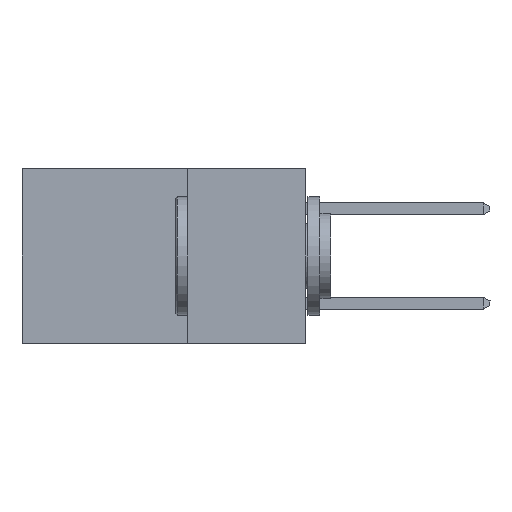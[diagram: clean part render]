
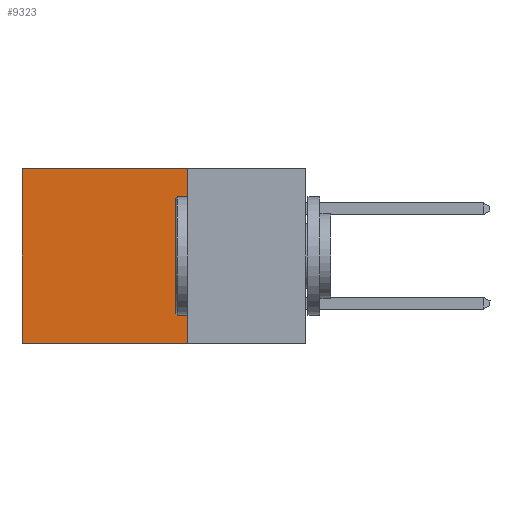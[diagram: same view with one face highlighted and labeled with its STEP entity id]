
A CAD part, left-side view. The second image highlights one B-rep face of the part: STEP entity #9323.
In plain terms, the highlighted planar face has unit normal (-1, 0, 0).
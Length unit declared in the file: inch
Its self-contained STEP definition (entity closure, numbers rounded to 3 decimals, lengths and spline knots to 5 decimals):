
#519 = LINE ( 'NONE', #17315, #11188 ) ;
#1501 = CARTESIAN_POINT ( 'NONE',  ( 0.298, 0.6, 0. ) ) ;
#3289 = CARTESIAN_POINT ( 'NONE',  ( 0.298, 0.25, 0. ) ) ;
#3666 = EDGE_CURVE ( 'NONE', #12631, #19099, #19870, .T. ) ;
#4229 = DIRECTION ( 'NONE',  ( 0., 1., 0. ) ) ;
#4754 = EDGE_CURVE ( 'NONE', #11919, #13870, #11239, .T. ) ;
#5230 = CARTESIAN_POINT ( 'NONE',  ( 0.298, 0.25, 0. ) ) ;
#5667 = FACE_OUTER_BOUND ( 'NONE', #6035, .T. ) ;
#5844 = CARTESIAN_POINT ( 'NONE',  ( 0.298, 0.6, -0.37 ) ) ;
#6035 = EDGE_LOOP ( 'NONE', ( #10221, #6075, #8414, #17358 ) ) ;
#6075 = ORIENTED_EDGE ( 'NONE', *, *, #6319, .F. ) ;
#6108 = DIRECTION ( 'NONE',  ( 0., 0., -1. ) ) ;
#6319 = EDGE_CURVE ( 'NONE', #19099, #13870, #519, .T. ) ;
#7981 = LINE ( 'NONE', #3289, #11563 ) ;
#8414 = ORIENTED_EDGE ( 'NONE', *, *, #3666, .F. ) ;
#9323 = ADVANCED_FACE ( 'NONE', ( #5667 ), #11535, .F. ) ;
#9333 = AXIS2_PLACEMENT_3D ( 'NONE', #5230, #13289, #18247 ) ;
#10035 = CARTESIAN_POINT ( 'NONE',  ( 0.298, 0.25, 0. ) ) ;
#10221 = ORIENTED_EDGE ( 'NONE', *, *, #4754, .T. ) ;
#10428 = VECTOR ( 'NONE', #17893, 39.37008 ) ;
#11188 = VECTOR ( 'NONE', #4229, 39.37008 ) ;
#11239 = LINE ( 'NONE', #1501, #10428 ) ;
#11535 = PLANE ( 'NONE',  #9333 ) ;
#11563 = VECTOR ( 'NONE', #18116, 39.37008 ) ;
#11919 = VERTEX_POINT ( 'NONE', #17958 ) ;
#12631 = VERTEX_POINT ( 'NONE', #10035 ) ;
#13289 = DIRECTION ( 'NONE',  ( 1., 0., 0. ) ) ;
#13870 = VERTEX_POINT ( 'NONE', #5844 ) ;
#15589 = CARTESIAN_POINT ( 'NONE',  ( 0.298, 0.25, -0.37 ) ) ;
#16639 = EDGE_CURVE ( 'NONE', #12631, #11919, #7981, .T. ) ;
#17315 = CARTESIAN_POINT ( 'NONE',  ( 0.298, 0.25, -0.37 ) ) ;
#17358 = ORIENTED_EDGE ( 'NONE', *, *, #16639, .T. ) ;
#17893 = DIRECTION ( 'NONE',  ( 0., 0., -1. ) ) ;
#17958 = CARTESIAN_POINT ( 'NONE',  ( 0.298, 0.6, 0. ) ) ;
#18116 = DIRECTION ( 'NONE',  ( 0., 1., 0. ) ) ;
#18247 = DIRECTION ( 'NONE',  ( 0., 0., -1. ) ) ;
#18611 = VECTOR ( 'NONE', #6108, 39.37008 ) ;
#18917 = CARTESIAN_POINT ( 'NONE',  ( 0.298, 0.25, 0. ) ) ;
#19099 = VERTEX_POINT ( 'NONE', #15589 ) ;
#19870 = LINE ( 'NONE', #18917, #18611 ) ;
